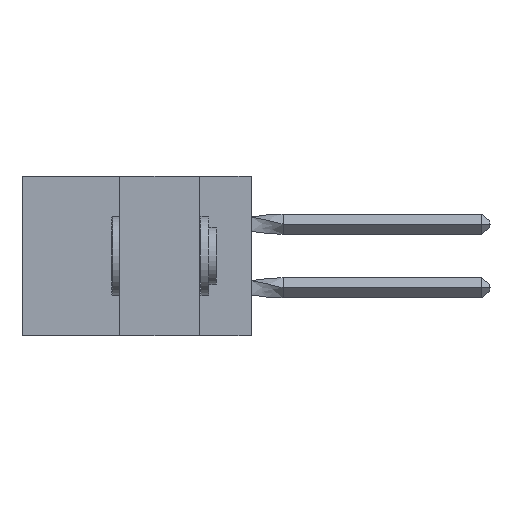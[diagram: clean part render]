
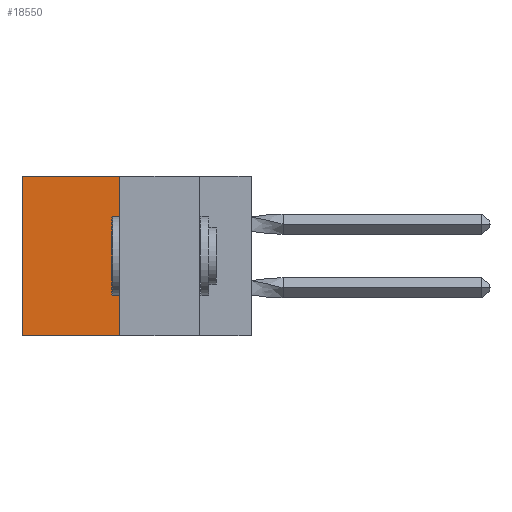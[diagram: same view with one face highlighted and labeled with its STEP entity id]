
A CAD part, left-side view. The second image highlights one B-rep face of the part: STEP entity #18550.
In plain terms, the highlighted planar face has unit normal (-1, 0, 0).
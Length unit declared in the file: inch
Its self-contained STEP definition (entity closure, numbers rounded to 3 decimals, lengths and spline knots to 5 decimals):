
#423 = LINE ( 'NONE', #8967, #22855 ) ;
#822 = CARTESIAN_POINT ( 'NONE',  ( 0.305, 0.72, 0. ) ) ;
#1516 = DIRECTION ( 'NONE',  ( 0., 0., -1. ) ) ;
#3273 = VECTOR ( 'NONE', #22485, 39.37008 ) ;
#4153 = FACE_OUTER_BOUND ( 'NONE', #16942, .T. ) ;
#5377 = AXIS2_PLACEMENT_3D ( 'NONE', #21067, #18690, #1516 ) ;
#6509 = ORIENTED_EDGE ( 'NONE', *, *, #20228, .F. ) ;
#8961 = DIRECTION ( 'NONE',  ( 0., 1., 0. ) ) ;
#8967 = CARTESIAN_POINT ( 'NONE',  ( 0.305, 0.413, 0. ) ) ;
#9619 = ORIENTED_EDGE ( 'NONE', *, *, #27687, .F. ) ;
#10924 = ORIENTED_EDGE ( 'NONE', *, *, #18598, .T. ) ;
#11338 = LINE ( 'NONE', #30359, #17468 ) ;
#11566 = DIRECTION ( 'NONE',  ( 0., 1., 0. ) ) ;
#12126 = VERTEX_POINT ( 'NONE', #25779 ) ;
#12129 = CARTESIAN_POINT ( 'NONE',  ( 0.305, 0.413, -0.5 ) ) ;
#12865 = VECTOR ( 'NONE', #8961, 39.37008 ) ;
#13081 = EDGE_CURVE ( 'NONE', #34535, #23660, #423, .T. ) ;
#16114 = ORIENTED_EDGE ( 'NONE', *, *, #13081, .T. ) ;
#16942 = EDGE_LOOP ( 'NONE', ( #10924, #6509, #9619, #16114 ) ) ;
#17468 = VECTOR ( 'NONE', #33226, 39.37008 ) ;
#18550 = ADVANCED_FACE ( 'NONE', ( #4153 ), #18576, .F. ) ;
#18576 = PLANE ( 'NONE',  #5377 ) ;
#18598 = EDGE_CURVE ( 'NONE', #23660, #12126, #19502, .T. ) ;
#18690 = DIRECTION ( 'NONE',  ( 1., 0., 0. ) ) ;
#19502 = LINE ( 'NONE', #30746, #3273 ) ;
#20228 = EDGE_CURVE ( 'NONE', #31707, #12126, #21648, .T. ) ;
#21067 = CARTESIAN_POINT ( 'NONE',  ( 0.305, 0.413, -0.5 ) ) ;
#21648 = LINE ( 'NONE', #28525, #12865 ) ;
#22485 = DIRECTION ( 'NONE',  ( 0., 0., -1. ) ) ;
#22855 = VECTOR ( 'NONE', #11566, 39.37008 ) ;
#23660 = VERTEX_POINT ( 'NONE', #822 ) ;
#25779 = CARTESIAN_POINT ( 'NONE',  ( 0.305, 0.72, -0.5 ) ) ;
#27687 = EDGE_CURVE ( 'NONE', #34535, #31707, #11338, .T. ) ;
#28525 = CARTESIAN_POINT ( 'NONE',  ( 0.305, 0.413, -0.5 ) ) ;
#29352 = CARTESIAN_POINT ( 'NONE',  ( 0.305, 0.413, 0. ) ) ;
#30359 = CARTESIAN_POINT ( 'NONE',  ( 0.305, 0.413, -0.5 ) ) ;
#30746 = CARTESIAN_POINT ( 'NONE',  ( 0.305, 0.72, -0.5 ) ) ;
#31707 = VERTEX_POINT ( 'NONE', #12129 ) ;
#33226 = DIRECTION ( 'NONE',  ( 0., 0., -1. ) ) ;
#34535 = VERTEX_POINT ( 'NONE', #29352 ) ;
